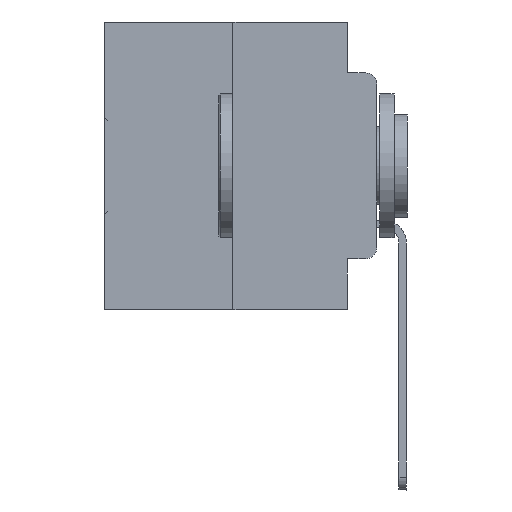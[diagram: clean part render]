
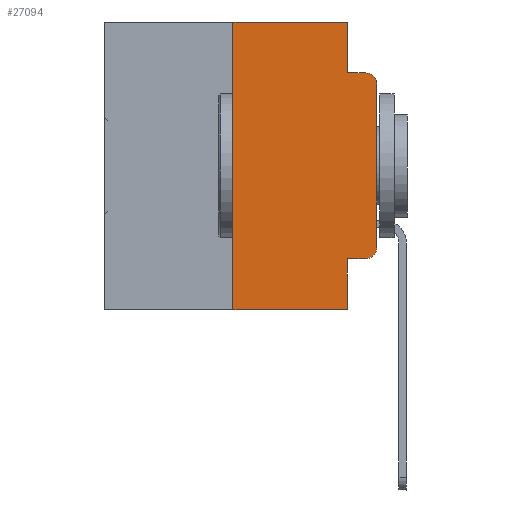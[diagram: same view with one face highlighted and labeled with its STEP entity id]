
A CAD part, left-side view. The second image highlights one B-rep face of the part: STEP entity #27094.
In plain terms, the highlighted planar face has unit normal (-1, 0, 0).
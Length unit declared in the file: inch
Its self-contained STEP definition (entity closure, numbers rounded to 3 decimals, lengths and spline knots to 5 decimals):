
#342 = CARTESIAN_POINT ( 'NONE',  ( 0., 0.051, -0.5 ) ) ;
#693 = ORIENTED_EDGE ( 'NONE', *, *, #28199, .F. ) ;
#1545 = DIRECTION ( 'NONE',  ( 0., 0., 1. ) ) ;
#2664 = CARTESIAN_POINT ( 'NONE',  ( 0., 0., -0.1085 ) ) ;
#2939 = CARTESIAN_POINT ( 'NONE',  ( 0., 0.25, 0. ) ) ;
#3375 = LINE ( 'NONE', #14283, #11538 ) ;
#3500 = CARTESIAN_POINT ( 'NONE',  ( 0., 0., -0.3915 ) ) ;
#3765 = ORIENTED_EDGE ( 'NONE', *, *, #16900, .T. ) ;
#3836 = FACE_OUTER_BOUND ( 'NONE', #30282, .T. ) ;
#4395 = AXIS2_PLACEMENT_3D ( 'NONE', #24897, #20050, #25116 ) ;
#4903 = DIRECTION ( 'NONE',  ( 0., -1., 0. ) ) ;
#5133 = VECTOR ( 'NONE', #1545, 39.37008 ) ;
#5389 = ORIENTED_EDGE ( 'NONE', *, *, #8231, .T. ) ;
#5734 = CARTESIAN_POINT ( 'NONE',  ( 0., 0.02, -0.4115 ) ) ;
#6204 = CARTESIAN_POINT ( 'NONE',  ( 0., 0.473, -0.5 ) ) ;
#7047 = CARTESIAN_POINT ( 'NONE',  ( 0., 0.473, 0. ) ) ;
#7301 = ORIENTED_EDGE ( 'NONE', *, *, #16547, .F. ) ;
#7411 = DIRECTION ( 'NONE',  ( 0., 0., -1. ) ) ;
#7452 = ORIENTED_EDGE ( 'NONE', *, *, #29655, .F. ) ;
#7832 = VERTEX_POINT ( 'NONE', #2664 ) ;
#8231 = EDGE_CURVE ( 'NONE', #22232, #10763, #20592, .T. ) ;
#8606 = VECTOR ( 'NONE', #17689, 39.37008 ) ;
#8918 = LINE ( 'NONE', #12158, #21936 ) ;
#8961 = CARTESIAN_POINT ( 'NONE',  ( 0., 0.051, -0.0885 ) ) ;
#10264 = LINE ( 'NONE', #7047, #8606 ) ;
#10763 = VERTEX_POINT ( 'NONE', #342 ) ;
#11159 = ORIENTED_EDGE ( 'NONE', *, *, #21085, .T. ) ;
#11246 = CARTESIAN_POINT ( 'NONE',  ( 0., 0.25, 0. ) ) ;
#11410 = LINE ( 'NONE', #11246, #19961 ) ;
#11538 = VECTOR ( 'NONE', #4903, 39.37008 ) ;
#12079 = LINE ( 'NONE', #30534, #5133 ) ;
#12158 = CARTESIAN_POINT ( 'NONE',  ( 0., 0.051, 0. ) ) ;
#12236 = PLANE ( 'NONE',  #17162 ) ;
#12582 = DIRECTION ( 'NONE',  ( -1., 0., 0. ) ) ;
#14283 = CARTESIAN_POINT ( 'NONE',  ( 0., 0.051, -0.4115 ) ) ;
#15026 = CARTESIAN_POINT ( 'NONE',  ( 0., 0.051, -0.0885 ) ) ;
#15127 = VERTEX_POINT ( 'NONE', #22657 ) ;
#15179 = EDGE_CURVE ( 'NONE', #29543, #22447, #10264, .T. ) ;
#16383 = EDGE_CURVE ( 'NONE', #22447, #26332, #8918, .T. ) ;
#16469 = DIRECTION ( 'NONE',  ( 0., -1., 0. ) ) ;
#16535 = ORIENTED_EDGE ( 'NONE', *, *, #21728, .T. ) ;
#16547 = EDGE_CURVE ( 'NONE', #26332, #32555, #18321, .T. ) ;
#16900 = EDGE_CURVE ( 'NONE', #7832, #32555, #21496, .T. ) ;
#17162 = AXIS2_PLACEMENT_3D ( 'NONE', #32286, #31850, #32428 ) ;
#17584 = CARTESIAN_POINT ( 'NONE',  ( 0., 0.02, -0.3915 ) ) ;
#17689 = DIRECTION ( 'NONE',  ( 0., -1., 0. ) ) ;
#18100 = CARTESIAN_POINT ( 'NONE',  ( 0., 0.051, 0. ) ) ;
#18178 = VERTEX_POINT ( 'NONE', #5734 ) ;
#18321 = LINE ( 'NONE', #8961, #30379 ) ;
#18527 = DIRECTION ( 'NONE',  ( 0., 0., -1. ) ) ;
#18890 = AXIS2_PLACEMENT_3D ( 'NONE', #17584, #12582, #7411 ) ;
#19214 = VECTOR ( 'NONE', #18527, 39.37008 ) ;
#19502 = EDGE_CURVE ( 'NONE', #27864, #7832, #12079, .T. ) ;
#19885 = DIRECTION ( 'NONE',  ( 0., 0., -1. ) ) ;
#19961 = VECTOR ( 'NONE', #27093, 39.37008 ) ;
#20050 = DIRECTION ( 'NONE',  ( -1., 0., 0. ) ) ;
#20592 = LINE ( 'NONE', #6204, #26605 ) ;
#21085 = EDGE_CURVE ( 'NONE', #15127, #18178, #3375, .T. ) ;
#21469 = CARTESIAN_POINT ( 'NONE',  ( 0., 0.051, 0. ) ) ;
#21496 = CIRCLE ( 'NONE', #4395, 0.02 ) ;
#21728 = EDGE_CURVE ( 'NONE', #18178, #27864, #28474, .T. ) ;
#21936 = VECTOR ( 'NONE', #19885, 39.37008 ) ;
#22232 = VERTEX_POINT ( 'NONE', #27859 ) ;
#22447 = VERTEX_POINT ( 'NONE', #21469 ) ;
#22657 = CARTESIAN_POINT ( 'NONE',  ( 0., 0.051, -0.4115 ) ) ;
#22872 = CARTESIAN_POINT ( 'NONE',  ( 0., 0.02, -0.0885 ) ) ;
#24255 = DIRECTION ( 'NONE',  ( 0., -1., 0. ) ) ;
#24897 = CARTESIAN_POINT ( 'NONE',  ( 0., 0.02, -0.1085 ) ) ;
#25116 = DIRECTION ( 'NONE',  ( 0., 0., -1. ) ) ;
#26088 = LINE ( 'NONE', #18100, #19214 ) ;
#26332 = VERTEX_POINT ( 'NONE', #15026 ) ;
#26605 = VECTOR ( 'NONE', #16469, 39.37008 ) ;
#27093 = DIRECTION ( 'NONE',  ( 0., 0., 1. ) ) ;
#27094 = ADVANCED_FACE ( 'NONE', ( #3836 ), #12236, .F. ) ;
#27489 = ORIENTED_EDGE ( 'NONE', *, *, #16383, .F. ) ;
#27859 = CARTESIAN_POINT ( 'NONE',  ( 0., 0.25, -0.5 ) ) ;
#27864 = VERTEX_POINT ( 'NONE', #3500 ) ;
#28199 = EDGE_CURVE ( 'NONE', #15127, #10763, #26088, .T. ) ;
#28474 = CIRCLE ( 'NONE', #18890, 0.02 ) ;
#28929 = ORIENTED_EDGE ( 'NONE', *, *, #19502, .T. ) ;
#29543 = VERTEX_POINT ( 'NONE', #2939 ) ;
#29655 = EDGE_CURVE ( 'NONE', #22232, #29543, #11410, .T. ) ;
#29768 = ORIENTED_EDGE ( 'NONE', *, *, #15179, .F. ) ;
#30282 = EDGE_LOOP ( 'NONE', ( #28929, #3765, #7301, #27489, #29768, #7452, #5389, #693, #11159, #16535 ) ) ;
#30379 = VECTOR ( 'NONE', #24255, 39.37008 ) ;
#30534 = CARTESIAN_POINT ( 'NONE',  ( 0., 0., 0. ) ) ;
#31850 = DIRECTION ( 'NONE',  ( 1., 0., 0. ) ) ;
#32286 = CARTESIAN_POINT ( 'NONE',  ( 0., 0.473, 0. ) ) ;
#32428 = DIRECTION ( 'NONE',  ( 0., 0., -1. ) ) ;
#32555 = VERTEX_POINT ( 'NONE', #22872 ) ;
